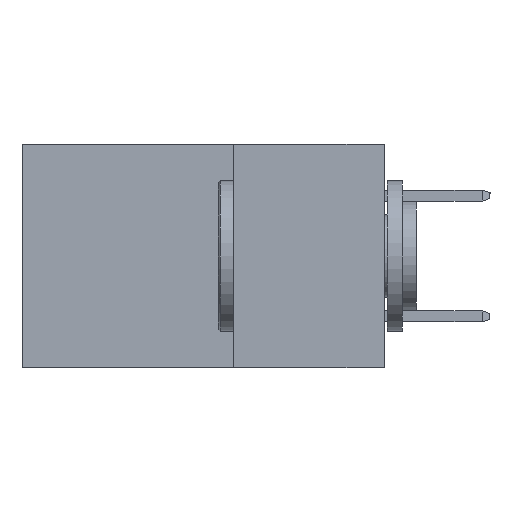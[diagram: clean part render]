
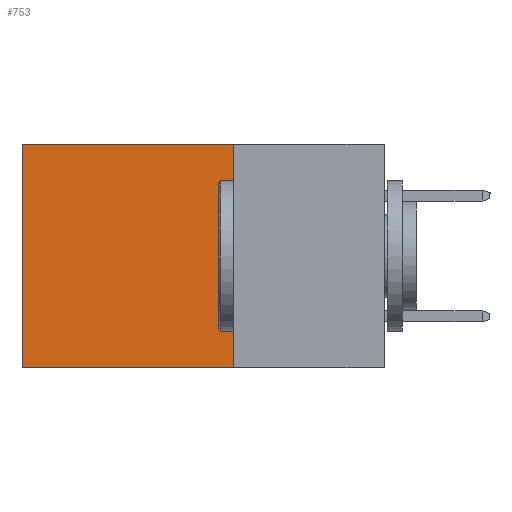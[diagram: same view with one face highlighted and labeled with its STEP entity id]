
A CAD part, left-side view. The second image highlights one B-rep face of the part: STEP entity #753.
In plain terms, the highlighted planar face has unit normal (-1, 0, 0).
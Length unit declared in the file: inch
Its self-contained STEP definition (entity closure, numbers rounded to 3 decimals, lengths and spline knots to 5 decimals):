
#133 = DIRECTION ( 'NONE',  ( 0., 0., -1. ) ) ;
#201 = DIRECTION ( 'NONE',  ( 1., 0., 0. ) ) ;
#372 = LINE ( 'NONE', #7316, #11309 ) ;
#538 = CARTESIAN_POINT ( 'NONE',  ( 0.2615, 0.25, 0. ) ) ;
#701 = ORIENTED_EDGE ( 'NONE', *, *, #12538, .F. ) ;
#753 = ADVANCED_FACE ( 'NONE', ( #7350 ), #9406, .F. ) ;
#1658 = VECTOR ( 'NONE', #10974, 39.37008 ) ;
#2520 = AXIS2_PLACEMENT_3D ( 'NONE', #10616, #201, #133 ) ;
#2898 = CARTESIAN_POINT ( 'NONE',  ( 0.2615, 0.6, -0.37 ) ) ;
#2918 = VECTOR ( 'NONE', #7847, 39.37008 ) ;
#3290 = EDGE_LOOP ( 'NONE', ( #3825, #701, #11284, #7410 ) ) ;
#3825 = ORIENTED_EDGE ( 'NONE', *, *, #6938, .T. ) ;
#3831 = VERTEX_POINT ( 'NONE', #9843 ) ;
#3892 = LINE ( 'NONE', #538, #8035 ) ;
#5660 = CARTESIAN_POINT ( 'NONE',  ( 0.2615, 0.25, -0.37 ) ) ;
#5796 = LINE ( 'NONE', #2898, #1658 ) ;
#6938 = EDGE_CURVE ( 'NONE', #3831, #7330, #5796, .T. ) ;
#7312 = VERTEX_POINT ( 'NONE', #9947 ) ;
#7316 = CARTESIAN_POINT ( 'NONE',  ( 0.2615, 0.25, -0.37 ) ) ;
#7330 = VERTEX_POINT ( 'NONE', #8942 ) ;
#7350 = FACE_OUTER_BOUND ( 'NONE', #3290, .T. ) ;
#7410 = ORIENTED_EDGE ( 'NONE', *, *, #9156, .T. ) ;
#7847 = DIRECTION ( 'NONE',  ( 0., 1., 0. ) ) ;
#7895 = DIRECTION ( 'NONE',  ( 0., 1., 0. ) ) ;
#8035 = VECTOR ( 'NONE', #7895, 39.37008 ) ;
#8942 = CARTESIAN_POINT ( 'NONE',  ( 0.2615, 0.6, -0.37 ) ) ;
#9156 = EDGE_CURVE ( 'NONE', #10094, #3831, #3892, .T. ) ;
#9406 = PLANE ( 'NONE',  #2520 ) ;
#9843 = CARTESIAN_POINT ( 'NONE',  ( 0.2615, 0.6, 0. ) ) ;
#9904 = EDGE_CURVE ( 'NONE', #10094, #7312, #372, .T. ) ;
#9947 = CARTESIAN_POINT ( 'NONE',  ( 0.2615, 0.25, -0.37 ) ) ;
#10094 = VERTEX_POINT ( 'NONE', #10480 ) ;
#10446 = DIRECTION ( 'NONE',  ( 0., 0., -1. ) ) ;
#10480 = CARTESIAN_POINT ( 'NONE',  ( 0.2615, 0.25, 0. ) ) ;
#10616 = CARTESIAN_POINT ( 'NONE',  ( 0.2615, 0.25, -0.37 ) ) ;
#10634 = LINE ( 'NONE', #5660, #2918 ) ;
#10974 = DIRECTION ( 'NONE',  ( 0., 0., -1. ) ) ;
#11284 = ORIENTED_EDGE ( 'NONE', *, *, #9904, .F. ) ;
#11309 = VECTOR ( 'NONE', #10446, 39.37008 ) ;
#12538 = EDGE_CURVE ( 'NONE', #7312, #7330, #10634, .T. ) ;
